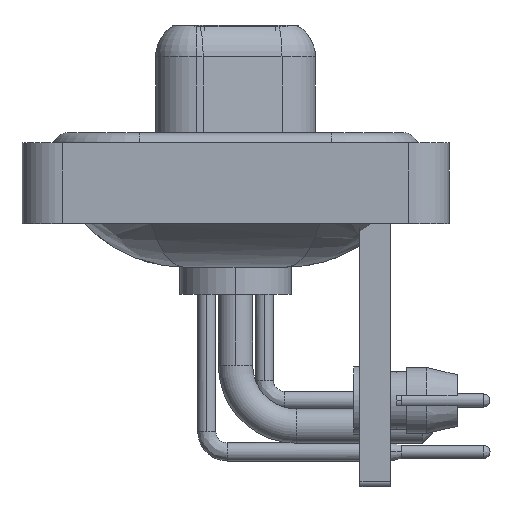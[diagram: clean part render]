
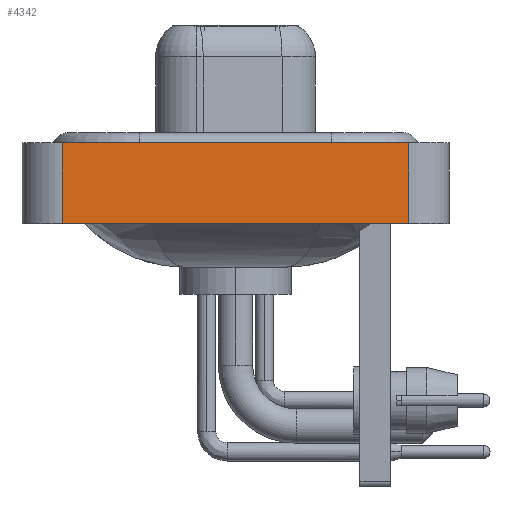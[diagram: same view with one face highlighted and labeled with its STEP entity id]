
A CAD part, left-side view. The second image highlights one B-rep face of the part: STEP entity #4342.
In plain terms, the highlighted planar face has unit normal (-1, 0, 0).
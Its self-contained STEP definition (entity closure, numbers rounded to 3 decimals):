
#255 = ORIENTED_EDGE ( 'NONE', *, *, #15531, .F. ) ;
#376 = PLANE ( 'NONE',  #1487 ) ;
#1487 = AXIS2_PLACEMENT_3D ( 'NONE', #8728, #17770, #4907 ) ;
#2918 = EDGE_CURVE ( 'NONE', #22327, #25099, #26682, .T. ) ;
#2992 = CARTESIAN_POINT ( 'NONE',  ( -7.35, -8.55, -3.6 ) ) ;
#3188 = EDGE_LOOP ( 'NONE', ( #25719, #255, #3411, #3302 ) ) ;
#3302 = ORIENTED_EDGE ( 'NONE', *, *, #8733, .T. ) ;
#3411 = ORIENTED_EDGE ( 'NONE', *, *, #4084, .F. ) ;
#3736 = VERTEX_POINT ( 'NONE', #4287 ) ;
#4084 = EDGE_CURVE ( 'NONE', #17404, #3736, #23218, .T. ) ;
#4287 = CARTESIAN_POINT ( 'NONE',  ( -7.35, 8.55, 0.4 ) ) ;
#4342 = ADVANCED_FACE ( 'NONE', ( #16678 ), #376, .T. ) ;
#4907 = DIRECTION ( 'NONE',  ( 0., 0., 1. ) ) ;
#7275 = LINE ( 'NONE', #26082, #24260 ) ;
#7517 = CARTESIAN_POINT ( 'NONE',  ( -7.35, 8.55, -3.6 ) ) ;
#7657 = DIRECTION ( 'NONE',  ( 0., 0., 1. ) ) ;
#7874 = CARTESIAN_POINT ( 'NONE',  ( -7.35, -8.55, -3.6 ) ) ;
#8018 = CARTESIAN_POINT ( 'NONE',  ( -7.35, -8.55, 0.4 ) ) ;
#8728 = CARTESIAN_POINT ( 'NONE',  ( -7.35, -8.55, -3.6 ) ) ;
#8733 = EDGE_CURVE ( 'NONE', #17404, #22327, #7275, .T. ) ;
#13707 = DIRECTION ( 'NONE',  ( 0., -1., 0. ) ) ;
#15531 = EDGE_CURVE ( 'NONE', #3736, #25099, #16513, .T. ) ;
#16513 = LINE ( 'NONE', #8018, #17555 ) ;
#16678 = FACE_OUTER_BOUND ( 'NONE', #3188, .T. ) ;
#17404 = VERTEX_POINT ( 'NONE', #25596 ) ;
#17555 = VECTOR ( 'NONE', #26964, 1000. ) ;
#17770 = DIRECTION ( 'NONE',  ( -1., 0., 0. ) ) ;
#19638 = CARTESIAN_POINT ( 'NONE',  ( -7.35, -8.55, 0.4 ) ) ;
#20725 = VECTOR ( 'NONE', #7657, 1000. ) ;
#21111 = VECTOR ( 'NONE', #22572, 1000. ) ;
#22327 = VERTEX_POINT ( 'NONE', #2992 ) ;
#22572 = DIRECTION ( 'NONE',  ( 0., 0., 1. ) ) ;
#23218 = LINE ( 'NONE', #7517, #20725 ) ;
#24260 = VECTOR ( 'NONE', #13707, 1000. ) ;
#25099 = VERTEX_POINT ( 'NONE', #19638 ) ;
#25596 = CARTESIAN_POINT ( 'NONE',  ( -7.35, 8.55, -3.6 ) ) ;
#25719 = ORIENTED_EDGE ( 'NONE', *, *, #2918, .T. ) ;
#26082 = CARTESIAN_POINT ( 'NONE',  ( -7.35, -8.55, -3.6 ) ) ;
#26682 = LINE ( 'NONE', #7874, #21111 ) ;
#26964 = DIRECTION ( 'NONE',  ( 0., -1., 0. ) ) ;
